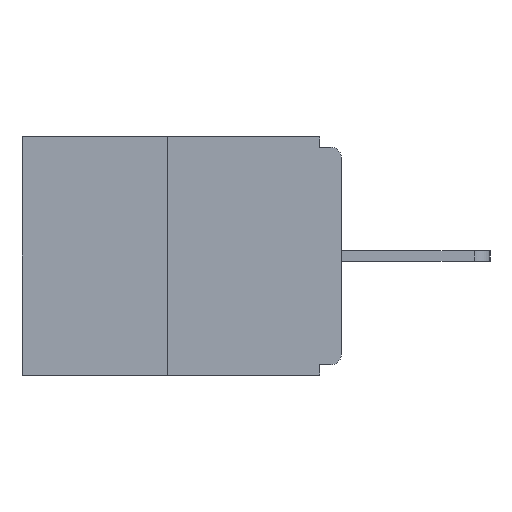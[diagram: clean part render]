
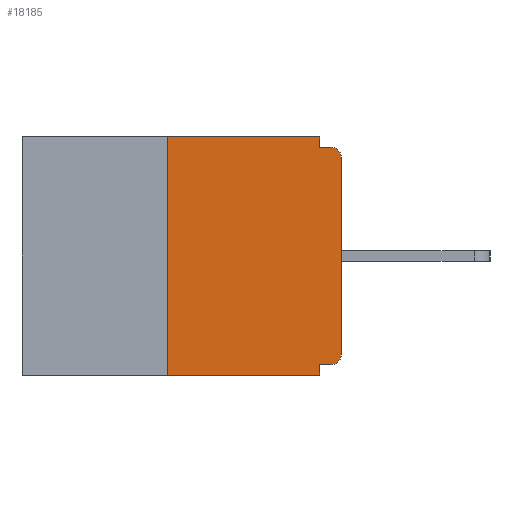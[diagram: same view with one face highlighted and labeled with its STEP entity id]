
A CAD part, left-side view. The second image highlights one B-rep face of the part: STEP entity #18185.
In plain terms, the highlighted planar face has unit normal (-1, 0, 0).
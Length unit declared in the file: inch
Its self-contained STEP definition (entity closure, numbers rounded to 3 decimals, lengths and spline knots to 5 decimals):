
#254 = CARTESIAN_POINT ( 'NONE',  ( 0., 0.25, 0. ) ) ;
#482 = ORIENTED_EDGE ( 'NONE', *, *, #16841, .F. ) ;
#939 = LINE ( 'NONE', #3226, #1385 ) ;
#999 = DIRECTION ( 'NONE',  ( 0., 0., -1. ) ) ;
#1385 = VECTOR ( 'NONE', #11672, 39.37008 ) ;
#1527 = CARTESIAN_POINT ( 'NONE',  ( 0., 0., 0. ) ) ;
#1671 = DIRECTION ( 'NONE',  ( 0., 0., -1. ) ) ;
#1721 = VERTEX_POINT ( 'NONE', #9539 ) ;
#1981 = EDGE_CURVE ( 'NONE', #15223, #10707, #4177, .T. ) ;
#2171 = CARTESIAN_POINT ( 'NONE',  ( 0., 0.031, -0.328 ) ) ;
#2311 = ORIENTED_EDGE ( 'NONE', *, *, #11240, .T. ) ;
#3077 = DIRECTION ( 'NONE',  ( 0., 0., 1. ) ) ;
#3163 = CARTESIAN_POINT ( 'NONE',  ( 0., 0., -0.328 ) ) ;
#3224 = EDGE_CURVE ( 'NONE', #8647, #13874, #6834, .T. ) ;
#3226 = CARTESIAN_POINT ( 'NONE',  ( 0., 0.031, 0. ) ) ;
#3337 = VECTOR ( 'NONE', #17162, 39.37008 ) ;
#3977 = AXIS2_PLACEMENT_3D ( 'NONE', #13019, #4550, #14422 ) ;
#4177 = LINE ( 'NONE', #8312, #7970 ) ;
#4201 = VERTEX_POINT ( 'NONE', #2171 ) ;
#4354 = LINE ( 'NONE', #12260, #6833 ) ;
#4550 = DIRECTION ( 'NONE',  ( -1., 0., 0. ) ) ;
#4787 = ORIENTED_EDGE ( 'NONE', *, *, #17996, .F. ) ;
#5142 = VECTOR ( 'NONE', #7449, 39.37008 ) ;
#5217 = CARTESIAN_POINT ( 'NONE',  ( 0., 0., -0.03 ) ) ;
#5287 = CARTESIAN_POINT ( 'NONE',  ( 0., 0.46, 0. ) ) ;
#6170 = ORIENTED_EDGE ( 'NONE', *, *, #1981, .F. ) ;
#6833 = VECTOR ( 'NONE', #13707, 39.37008 ) ;
#6834 = LINE ( 'NONE', #1527, #13417 ) ;
#6939 = LINE ( 'NONE', #5287, #14389 ) ;
#7169 = CARTESIAN_POINT ( 'NONE',  ( 0., 0.031, 0. ) ) ;
#7171 = EDGE_CURVE ( 'NONE', #15979, #8647, #17587, .T. ) ;
#7449 = DIRECTION ( 'NONE',  ( 0., 0., 1. ) ) ;
#7926 = VECTOR ( 'NONE', #1671, 39.37008 ) ;
#7970 = VECTOR ( 'NONE', #18212, 39.37008 ) ;
#8094 = DIRECTION ( 'NONE',  ( 0., -1., 0. ) ) ;
#8179 = CARTESIAN_POINT ( 'NONE',  ( 0., 0.015, -0.03 ) ) ;
#8232 = VERTEX_POINT ( 'NONE', #12522 ) ;
#8312 = CARTESIAN_POINT ( 'NONE',  ( 0., 0., -0.015 ) ) ;
#8385 = LINE ( 'NONE', #13053, #7926 ) ;
#8647 = VERTEX_POINT ( 'NONE', #10920 ) ;
#9458 = ORIENTED_EDGE ( 'NONE', *, *, #7171, .T. ) ;
#9488 = AXIS2_PLACEMENT_3D ( 'NONE', #8179, #17881, #9572 ) ;
#9539 = CARTESIAN_POINT ( 'NONE',  ( 0., 0.031, -0.343 ) ) ;
#9552 = DIRECTION ( 'NONE',  ( 1., 0., 0. ) ) ;
#9572 = DIRECTION ( 'NONE',  ( 0., 0., -1. ) ) ;
#10316 = EDGE_CURVE ( 'NONE', #4201, #1721, #8385, .T. ) ;
#10330 = ORIENTED_EDGE ( 'NONE', *, *, #11566, .F. ) ;
#10539 = CIRCLE ( 'NONE', #9488, 0.015 ) ;
#10707 = VERTEX_POINT ( 'NONE', #11046 ) ;
#10920 = CARTESIAN_POINT ( 'NONE',  ( 0., 0., -0.313 ) ) ;
#11046 = CARTESIAN_POINT ( 'NONE',  ( 0., 0.015, -0.015 ) ) ;
#11214 = EDGE_CURVE ( 'NONE', #8232, #1721, #4354, .T. ) ;
#11240 = EDGE_CURVE ( 'NONE', #13874, #10707, #10539, .T. ) ;
#11566 = EDGE_CURVE ( 'NONE', #13501, #15223, #939, .T. ) ;
#11672 = DIRECTION ( 'NONE',  ( 0., 0., -1. ) ) ;
#11771 = VERTEX_POINT ( 'NONE', #17691 ) ;
#11828 = ORIENTED_EDGE ( 'NONE', *, *, #11214, .T. ) ;
#12260 = CARTESIAN_POINT ( 'NONE',  ( 0., 0.46, -0.343 ) ) ;
#12272 = AXIS2_PLACEMENT_3D ( 'NONE', #17866, #9552, #999 ) ;
#12522 = CARTESIAN_POINT ( 'NONE',  ( 0., 0.25, -0.343 ) ) ;
#13019 = CARTESIAN_POINT ( 'NONE',  ( 0., 0.015, -0.313 ) ) ;
#13053 = CARTESIAN_POINT ( 'NONE',  ( 0., 0.031, -0.343 ) ) ;
#13201 = ORIENTED_EDGE ( 'NONE', *, *, #3224, .T. ) ;
#13417 = VECTOR ( 'NONE', #3077, 39.37008 ) ;
#13501 = VERTEX_POINT ( 'NONE', #7169 ) ;
#13707 = DIRECTION ( 'NONE',  ( 0., -1., 0. ) ) ;
#13874 = VERTEX_POINT ( 'NONE', #5217 ) ;
#13953 = FACE_OUTER_BOUND ( 'NONE', #16339, .T. ) ;
#13986 = CARTESIAN_POINT ( 'NONE',  ( 0., 0.031, -0.015 ) ) ;
#14389 = VECTOR ( 'NONE', #8094, 39.37008 ) ;
#14422 = DIRECTION ( 'NONE',  ( 0., 0., -1. ) ) ;
#14611 = LINE ( 'NONE', #3163, #3337 ) ;
#15183 = ORIENTED_EDGE ( 'NONE', *, *, #18175, .F. ) ;
#15223 = VERTEX_POINT ( 'NONE', #13986 ) ;
#15608 = ORIENTED_EDGE ( 'NONE', *, *, #10316, .F. ) ;
#15979 = VERTEX_POINT ( 'NONE', #16686 ) ;
#16339 = EDGE_LOOP ( 'NONE', ( #15183, #482, #11828, #15608, #4787, #9458, #13201, #2311, #6170, #10330 ) ) ;
#16338 = LINE ( 'NONE', #254, #5142 ) ;
#16440 = PLANE ( 'NONE',  #12272 ) ;
#16686 = CARTESIAN_POINT ( 'NONE',  ( 0., 0.015, -0.328 ) ) ;
#16841 = EDGE_CURVE ( 'NONE', #8232, #11771, #16338, .T. ) ;
#17162 = DIRECTION ( 'NONE',  ( 0., 1., 0. ) ) ;
#17587 = CIRCLE ( 'NONE', #3977, 0.015 ) ;
#17691 = CARTESIAN_POINT ( 'NONE',  ( 0., 0.25, 0. ) ) ;
#17866 = CARTESIAN_POINT ( 'NONE',  ( 0., 0.46, 0. ) ) ;
#17881 = DIRECTION ( 'NONE',  ( -1., 0., 0. ) ) ;
#17996 = EDGE_CURVE ( 'NONE', #15979, #4201, #14611, .T. ) ;
#18175 = EDGE_CURVE ( 'NONE', #11771, #13501, #6939, .T. ) ;
#18185 = ADVANCED_FACE ( 'NONE', ( #13953 ), #16440, .F. ) ;
#18212 = DIRECTION ( 'NONE',  ( 0., -1., 0. ) ) ;
